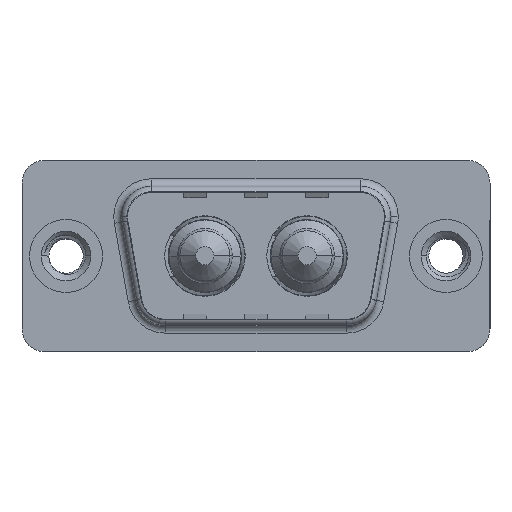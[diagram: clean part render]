
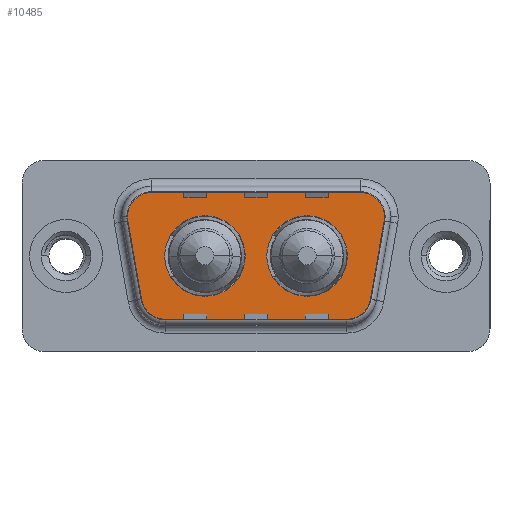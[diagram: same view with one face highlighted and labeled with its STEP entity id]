
A CAD part, top view. The second image highlights one B-rep face of the part: STEP entity #10485.
In plain terms, the highlighted planar face has unit normal (0, 0, 1).
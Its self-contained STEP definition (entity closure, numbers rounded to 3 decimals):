
#31 = CARTESIAN_POINT ( 'NONE',  ( 20.511, -3.247, 0. ) ) ;
#57 = VECTOR ( 'NONE', #7647, 1000. ) ;
#203 = AXIS2_PLACEMENT_3D ( 'NONE', #10435, #1798, #405 ) ;
#405 = DIRECTION ( 'NONE',  ( 1., 0., 0. ) ) ;
#430 = CIRCLE ( 'NONE', #7652, 2.65 ) ;
#460 = DIRECTION ( 'NONE',  ( 1., 0., 0. ) ) ;
#577 = EDGE_CURVE ( 'NONE', #9116, #4204, #15742, .T. ) ;
#708 = CARTESIAN_POINT ( 'NONE',  ( 18.541, -4.9, 0. ) ) ;
#766 = VERTEX_POINT ( 'NONE', #9150 ) ;
#1443 = FACE_BOUND ( 'NONE', #3066, .T. ) ;
#1558 = CARTESIAN_POINT ( 'NONE',  ( 3.466, 2.553, 0. ) ) ;
#1685 = EDGE_LOOP ( 'NONE', ( #4935, #5348 ) ) ;
#1786 = VECTOR ( 'NONE', #4558, 1000. ) ;
#1798 = DIRECTION ( 'NONE',  ( 0., 0., 1. ) ) ;
#1871 = VERTEX_POINT ( 'NONE', #12602 ) ;
#2096 = CARTESIAN_POINT ( 'NONE',  ( 19.564, 2.9, 0. ) ) ;
#2208 = CIRCLE ( 'NONE', #203, 2.65 ) ;
#2230 = DIRECTION ( 'NONE',  ( 0., 0., 1. ) ) ;
#2361 = AXIS2_PLACEMENT_3D ( 'NONE', #12201, #4949, #13410 ) ;
#2568 = EDGE_CURVE ( 'NONE', #4237, #12091, #9078, .T. ) ;
#2667 = ORIENTED_EDGE ( 'NONE', *, *, #577, .T. ) ;
#2785 = CIRCLE ( 'NONE', #8008, 2. ) ;
#3019 = ORIENTED_EDGE ( 'NONE', *, *, #14190, .F. ) ;
#3066 = EDGE_LOOP ( 'NONE', ( #3019, #14688 ) ) ;
#3094 = VERTEX_POINT ( 'NONE', #31 ) ;
#3175 = AXIS2_PLACEMENT_3D ( 'NONE', #3938, #5011, #9930 ) ;
#3274 = CARTESIAN_POINT ( 'NONE',  ( 15.86, 0., 0. ) ) ;
#3318 = CIRCLE ( 'NONE', #5830, 2. ) ;
#3327 = EDGE_CURVE ( 'NONE', #766, #13770, #2208, .T. ) ;
#3382 = EDGE_CURVE ( 'NONE', #7857, #4237, #11151, .T. ) ;
#3648 = AXIS2_PLACEMENT_3D ( 'NONE', #9567, #9516, #14612 ) ;
#3700 = EDGE_CURVE ( 'NONE', #6305, #5666, #7363, .T. ) ;
#3938 = CARTESIAN_POINT ( 'NONE',  ( 5.436, 2.9, 0. ) ) ;
#4049 = CARTESIAN_POINT ( 'NONE',  ( 5.436, 4.9, 0. ) ) ;
#4083 = CARTESIAN_POINT ( 'NONE',  ( 4.489, -3.247, 0. ) ) ;
#4204 = VERTEX_POINT ( 'NONE', #708 ) ;
#4237 = VERTEX_POINT ( 'NONE', #7768 ) ;
#4504 = CARTESIAN_POINT ( 'NONE',  ( 6.459, -2.9, 0. ) ) ;
#4527 = DIRECTION ( 'NONE',  ( 1., 0., 0. ) ) ;
#4558 = DIRECTION ( 'NONE',  ( 0.174, 0.985, 0. ) ) ;
#4707 = VECTOR ( 'NONE', #11326, 1000. ) ;
#4904 = AXIS2_PLACEMENT_3D ( 'NONE', #13474, #6205, #14700 ) ;
#4935 = ORIENTED_EDGE ( 'NONE', *, *, #7387, .F. ) ;
#4949 = DIRECTION ( 'NONE',  ( 0., 0., 1. ) ) ;
#4962 = ORIENTED_EDGE ( 'NONE', *, *, #12147, .T. ) ;
#5011 = DIRECTION ( 'NONE',  ( 0., 0., 1. ) ) ;
#5058 = LINE ( 'NONE', #13039, #1786 ) ;
#5203 = AXIS2_PLACEMENT_3D ( 'NONE', #6795, #15286, #8010 ) ;
#5220 = CARTESIAN_POINT ( 'NONE',  ( 6.459, -4.9, 0. ) ) ;
#5225 = VERTEX_POINT ( 'NONE', #8914 ) ;
#5348 = ORIENTED_EDGE ( 'NONE', *, *, #7116, .F. ) ;
#5480 = FACE_OUTER_BOUND ( 'NONE', #14159, .T. ) ;
#5666 = VERTEX_POINT ( 'NONE', #5705 ) ;
#5705 = CARTESIAN_POINT ( 'NONE',  ( 3.466, 2.553, 0. ) ) ;
#5716 = DIRECTION ( 'NONE',  ( -1., 0., 0. ) ) ;
#5722 = CARTESIAN_POINT ( 'NONE',  ( 21.534, 2.553, 0. ) ) ;
#5830 = AXIS2_PLACEMENT_3D ( 'NONE', #4504, #12978, #5716 ) ;
#6045 = CIRCLE ( 'NONE', #4904, 2.65 ) ;
#6205 = DIRECTION ( 'NONE',  ( 0., 0., 1. ) ) ;
#6226 = CARTESIAN_POINT ( 'NONE',  ( 18.51, 0., 0. ) ) ;
#6305 = VERTEX_POINT ( 'NONE', #11493 ) ;
#6705 = PLANE ( 'NONE',  #2361 ) ;
#6795 = CARTESIAN_POINT ( 'NONE',  ( 9.14, 0., 0. ) ) ;
#7116 = EDGE_CURVE ( 'NONE', #5225, #1871, #11930, .T. ) ;
#7363 = CIRCLE ( 'NONE', #3175, 2. ) ;
#7387 = EDGE_CURVE ( 'NONE', #1871, #5225, #6045, .T. ) ;
#7488 = ORIENTED_EDGE ( 'NONE', *, *, #11019, .T. ) ;
#7577 = AXIS2_PLACEMENT_3D ( 'NONE', #2096, #10075, #10153 ) ;
#7631 = VERTEX_POINT ( 'NONE', #4083 ) ;
#7647 = DIRECTION ( 'NONE',  ( 0.174, -0.985, 0. ) ) ;
#7652 = AXIS2_PLACEMENT_3D ( 'NONE', #3274, #11775, #4527 ) ;
#7768 = CARTESIAN_POINT ( 'NONE',  ( 21.564, 2.9, 0. ) ) ;
#7857 = VERTEX_POINT ( 'NONE', #5722 ) ;
#7924 = FACE_BOUND ( 'NONE', #1685, .T. ) ;
#8008 = AXIS2_PLACEMENT_3D ( 'NONE', #9530, #2230, #10734 ) ;
#8010 = DIRECTION ( 'NONE',  ( 1., 0., 0. ) ) ;
#8320 = ORIENTED_EDGE ( 'NONE', *, *, #3700, .T. ) ;
#8914 = CARTESIAN_POINT ( 'NONE',  ( 6.49, 0., 0. ) ) ;
#8981 = ORIENTED_EDGE ( 'NONE', *, *, #9088, .T. ) ;
#9038 = EDGE_CURVE ( 'NONE', #7631, #9116, #3318, .T. ) ;
#9078 = CIRCLE ( 'NONE', #3648, 2. ) ;
#9088 = EDGE_CURVE ( 'NONE', #3094, #7857, #5058, .T. ) ;
#9116 = VERTEX_POINT ( 'NONE', #11863 ) ;
#9150 = CARTESIAN_POINT ( 'NONE',  ( 13.21, 0., 0. ) ) ;
#9418 = LINE ( 'NONE', #1558, #57 ) ;
#9516 = DIRECTION ( 'NONE',  ( 0., 0., 1. ) ) ;
#9530 = CARTESIAN_POINT ( 'NONE',  ( 18.541, -2.9, 0. ) ) ;
#9567 = CARTESIAN_POINT ( 'NONE',  ( 19.564, 2.9, 0. ) ) ;
#9930 = DIRECTION ( 'NONE',  ( 1., 0., 0. ) ) ;
#10075 = DIRECTION ( 'NONE',  ( 0., 0., 1. ) ) ;
#10153 = DIRECTION ( 'NONE',  ( -1., 0., 0. ) ) ;
#10435 = CARTESIAN_POINT ( 'NONE',  ( 15.86, 0., 0. ) ) ;
#10439 = ORIENTED_EDGE ( 'NONE', *, *, #3382, .T. ) ;
#10485 = ADVANCED_FACE ( 'NONE', ( #1443, #7924, #5480 ), #6705, .T. ) ;
#10677 = EDGE_CURVE ( 'NONE', #4204, #3094, #2785, .T. ) ;
#10734 = DIRECTION ( 'NONE',  ( 1., 0., 0. ) ) ;
#11019 = EDGE_CURVE ( 'NONE', #12091, #6305, #11141, .T. ) ;
#11141 = LINE ( 'NONE', #4049, #4707 ) ;
#11151 = CIRCLE ( 'NONE', #7577, 2. ) ;
#11326 = DIRECTION ( 'NONE',  ( -1., 0., 0. ) ) ;
#11493 = CARTESIAN_POINT ( 'NONE',  ( 5.436, 4.9, 0. ) ) ;
#11582 = ORIENTED_EDGE ( 'NONE', *, *, #9038, .T. ) ;
#11775 = DIRECTION ( 'NONE',  ( 0., 0., 1. ) ) ;
#11863 = CARTESIAN_POINT ( 'NONE',  ( 6.459, -4.9, 0. ) ) ;
#11930 = CIRCLE ( 'NONE', #5203, 2.65 ) ;
#12040 = CARTESIAN_POINT ( 'NONE',  ( 19.564, 4.9, 0. ) ) ;
#12091 = VERTEX_POINT ( 'NONE', #12040 ) ;
#12147 = EDGE_CURVE ( 'NONE', #5666, #7631, #9418, .T. ) ;
#12201 = CARTESIAN_POINT ( 'NONE',  ( 18.541, -2.9, 0. ) ) ;
#12532 = VECTOR ( 'NONE', #460, 1000. ) ;
#12602 = CARTESIAN_POINT ( 'NONE',  ( 11.79, 0., 0. ) ) ;
#12978 = DIRECTION ( 'NONE',  ( 0., 0., 1. ) ) ;
#13039 = CARTESIAN_POINT ( 'NONE',  ( 21.534, 2.553, 0. ) ) ;
#13410 = DIRECTION ( 'NONE',  ( 1., 0., 0. ) ) ;
#13474 = CARTESIAN_POINT ( 'NONE',  ( 9.14, 0., 0. ) ) ;
#13770 = VERTEX_POINT ( 'NONE', #6226 ) ;
#13815 = ORIENTED_EDGE ( 'NONE', *, *, #2568, .T. ) ;
#14122 = ORIENTED_EDGE ( 'NONE', *, *, #10677, .T. ) ;
#14159 = EDGE_LOOP ( 'NONE', ( #14122, #8981, #10439, #13815, #7488, #8320, #4962, #11582, #2667 ) ) ;
#14190 = EDGE_CURVE ( 'NONE', #13770, #766, #430, .T. ) ;
#14612 = DIRECTION ( 'NONE',  ( -1., 0., 0. ) ) ;
#14688 = ORIENTED_EDGE ( 'NONE', *, *, #3327, .F. ) ;
#14700 = DIRECTION ( 'NONE',  ( 1., 0., 0. ) ) ;
#15286 = DIRECTION ( 'NONE',  ( 0., 0., 1. ) ) ;
#15742 = LINE ( 'NONE', #5220, #12532 ) ;
